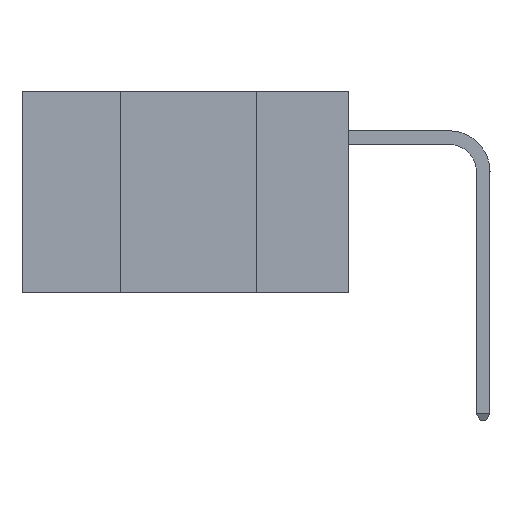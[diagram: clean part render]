
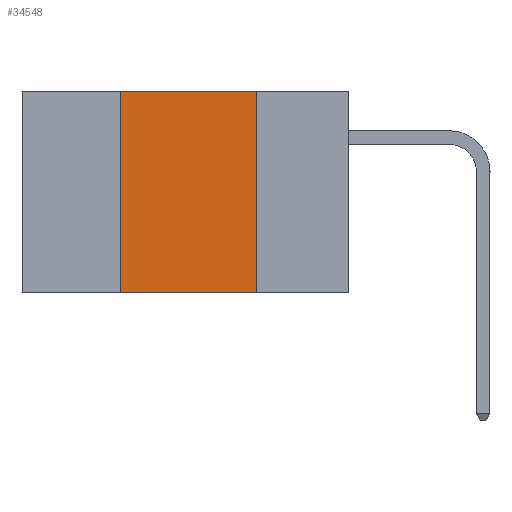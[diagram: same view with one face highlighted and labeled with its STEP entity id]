
A CAD part, left-side view. The second image highlights one B-rep face of the part: STEP entity #34548.
In plain terms, the highlighted planar face has unit normal (-1, 0, 0).
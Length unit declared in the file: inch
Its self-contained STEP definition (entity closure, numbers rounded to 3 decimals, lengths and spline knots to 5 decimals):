
#256 = CARTESIAN_POINT ( 'NONE',  ( 0., 0.17, 0. ) ) ;
#1150 = ORIENTED_EDGE ( 'NONE', *, *, #3740, .F. ) ;
#3740 = EDGE_CURVE ( 'NONE', #32837, #27309, #24327, .T. ) ;
#4477 = EDGE_CURVE ( 'NONE', #11058, #32837, #35676, .T. ) ;
#7112 = DIRECTION ( 'NONE',  ( 0., 0., -1. ) ) ;
#7430 = FACE_OUTER_BOUND ( 'NONE', #13564, .T. ) ;
#7609 = VECTOR ( 'NONE', #16754, 39.37008 ) ;
#7790 = DIRECTION ( 'NONE',  ( 0., 0., -1. ) ) ;
#10317 = DIRECTION ( 'NONE',  ( 0., 0., 1. ) ) ;
#10570 = ORIENTED_EDGE ( 'NONE', *, *, #4477, .F. ) ;
#11058 = VERTEX_POINT ( 'NONE', #32093 ) ;
#11365 = VECTOR ( 'NONE', #10317, 39.37008 ) ;
#13345 = DIRECTION ( 'NONE',  ( 1., 0., 0. ) ) ;
#13564 = EDGE_LOOP ( 'NONE', ( #30745, #1150, #10570, #14035 ) ) ;
#14035 = ORIENTED_EDGE ( 'NONE', *, *, #33680, .T. ) ;
#16029 = VECTOR ( 'NONE', #32312, 39.37008 ) ;
#16665 = CARTESIAN_POINT ( 'NONE',  ( 0., 0.6, 0. ) ) ;
#16754 = DIRECTION ( 'NONE',  ( 0., -1., 0. ) ) ;
#21407 = CARTESIAN_POINT ( 'NONE',  ( 0., 0.42, 0. ) ) ;
#23089 = EDGE_CURVE ( 'NONE', #27309, #23939, #32662, .T. ) ;
#23125 = CARTESIAN_POINT ( 'NONE',  ( 0., 0.17, -0.37 ) ) ;
#23939 = VERTEX_POINT ( 'NONE', #23125 ) ;
#24132 = CARTESIAN_POINT ( 'NONE',  ( 0., 0.17, 0. ) ) ;
#24327 = LINE ( 'NONE', #35628, #16029 ) ;
#24733 = LINE ( 'NONE', #30485, #7609 ) ;
#27309 = VERTEX_POINT ( 'NONE', #256 ) ;
#30056 = CARTESIAN_POINT ( 'NONE',  ( 0., 0.42, 0. ) ) ;
#30485 = CARTESIAN_POINT ( 'NONE',  ( 0., 0.6, -0.37 ) ) ;
#30745 = ORIENTED_EDGE ( 'NONE', *, *, #23089, .F. ) ;
#30754 = PLANE ( 'NONE',  #35953 ) ;
#32093 = CARTESIAN_POINT ( 'NONE',  ( 0., 0.42, -0.37 ) ) ;
#32312 = DIRECTION ( 'NONE',  ( 0., -1., 0. ) ) ;
#32662 = LINE ( 'NONE', #24132, #34419 ) ;
#32837 = VERTEX_POINT ( 'NONE', #30056 ) ;
#33680 = EDGE_CURVE ( 'NONE', #11058, #23939, #24733, .T. ) ;
#34419 = VECTOR ( 'NONE', #7112, 39.37008 ) ;
#34548 = ADVANCED_FACE ( 'NONE', ( #7430 ), #30754, .F. ) ;
#35628 = CARTESIAN_POINT ( 'NONE',  ( 0., 0.6, 0. ) ) ;
#35676 = LINE ( 'NONE', #21407, #11365 ) ;
#35953 = AXIS2_PLACEMENT_3D ( 'NONE', #16665, #13345, #7790 ) ;
